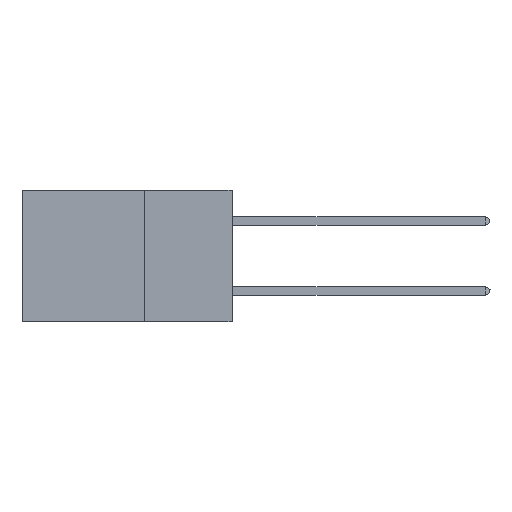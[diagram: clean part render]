
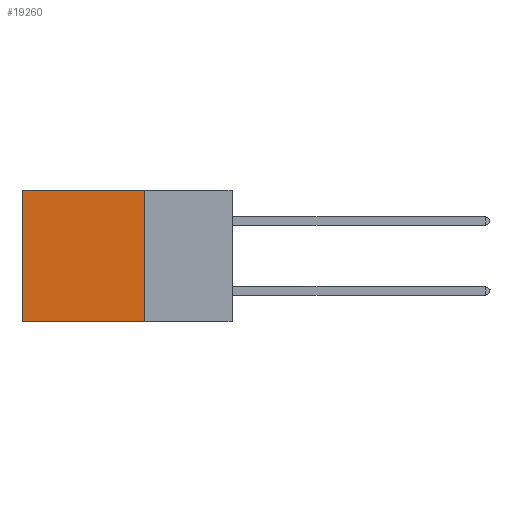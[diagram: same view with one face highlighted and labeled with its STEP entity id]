
A CAD part, left-side view. The second image highlights one B-rep face of the part: STEP entity #19260.
In plain terms, the highlighted planar face has unit normal (-1, 0, 0).
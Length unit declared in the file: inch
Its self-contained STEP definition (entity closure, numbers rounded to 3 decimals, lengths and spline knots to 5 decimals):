
#564 = EDGE_CURVE ( 'NONE', #13091, #6818, #5676, .T. ) ;
#1779 = DIRECTION ( 'NONE',  ( 0., 0., -1. ) ) ;
#1872 = CARTESIAN_POINT ( 'NONE',  ( 0.2875, 0.6, 0. ) ) ;
#2413 = FACE_OUTER_BOUND ( 'NONE', #7523, .T. ) ;
#2465 = CARTESIAN_POINT ( 'NONE',  ( 0.2875, 0.25, -0.375 ) ) ;
#4401 = CARTESIAN_POINT ( 'NONE',  ( 0.2875, 0.25, -0.375 ) ) ;
#4817 = CARTESIAN_POINT ( 'NONE',  ( 0.2875, 0.6, -0.375 ) ) ;
#5191 = VECTOR ( 'NONE', #16277, 39.37008 ) ;
#5263 = CARTESIAN_POINT ( 'NONE',  ( 0.2875, 0.25, -0.375 ) ) ;
#5676 = LINE ( 'NONE', #7004, #5191 ) ;
#5743 = VECTOR ( 'NONE', #9903, 39.37008 ) ;
#6146 = ORIENTED_EDGE ( 'NONE', *, *, #14423, .F. ) ;
#6818 = VERTEX_POINT ( 'NONE', #5263 ) ;
#7004 = CARTESIAN_POINT ( 'NONE',  ( 0.2875, 0.25, -0.375 ) ) ;
#7523 = EDGE_LOOP ( 'NONE', ( #11580, #6146, #19399, #19887 ) ) ;
#7527 = DIRECTION ( 'NONE',  ( 0., 0., -1. ) ) ;
#7691 = EDGE_CURVE ( 'NONE', #13410, #8616, #9154, .T. ) ;
#8616 = VERTEX_POINT ( 'NONE', #18755 ) ;
#9062 = LINE ( 'NONE', #2465, #13911 ) ;
#9154 = LINE ( 'NONE', #4817, #14975 ) ;
#9903 = DIRECTION ( 'NONE',  ( 0., 1., 0. ) ) ;
#10401 = CARTESIAN_POINT ( 'NONE',  ( 0.2875, 0.25, 0. ) ) ;
#11254 = EDGE_CURVE ( 'NONE', #13091, #13410, #18833, .T. ) ;
#11580 = ORIENTED_EDGE ( 'NONE', *, *, #7691, .T. ) ;
#13091 = VERTEX_POINT ( 'NONE', #10401 ) ;
#13147 = DIRECTION ( 'NONE',  ( 0., 1., 0. ) ) ;
#13410 = VERTEX_POINT ( 'NONE', #1872 ) ;
#13911 = VECTOR ( 'NONE', #13147, 39.37008 ) ;
#14061 = AXIS2_PLACEMENT_3D ( 'NONE', #4401, #16773, #7527 ) ;
#14423 = EDGE_CURVE ( 'NONE', #6818, #8616, #9062, .T. ) ;
#14555 = CARTESIAN_POINT ( 'NONE',  ( 0.2875, 0.25, 0. ) ) ;
#14975 = VECTOR ( 'NONE', #1779, 39.37008 ) ;
#16277 = DIRECTION ( 'NONE',  ( 0., 0., -1. ) ) ;
#16653 = PLANE ( 'NONE',  #14061 ) ;
#16773 = DIRECTION ( 'NONE',  ( 1., 0., 0. ) ) ;
#18755 = CARTESIAN_POINT ( 'NONE',  ( 0.2875, 0.6, -0.375 ) ) ;
#18833 = LINE ( 'NONE', #14555, #5743 ) ;
#19260 = ADVANCED_FACE ( 'NONE', ( #2413 ), #16653, .F. ) ;
#19399 = ORIENTED_EDGE ( 'NONE', *, *, #564, .F. ) ;
#19887 = ORIENTED_EDGE ( 'NONE', *, *, #11254, .T. ) ;
